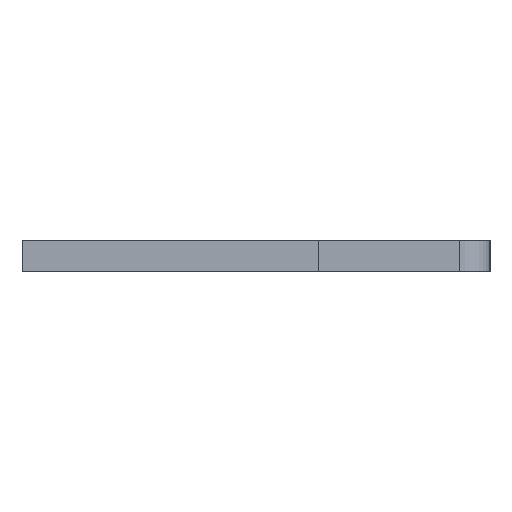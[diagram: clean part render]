
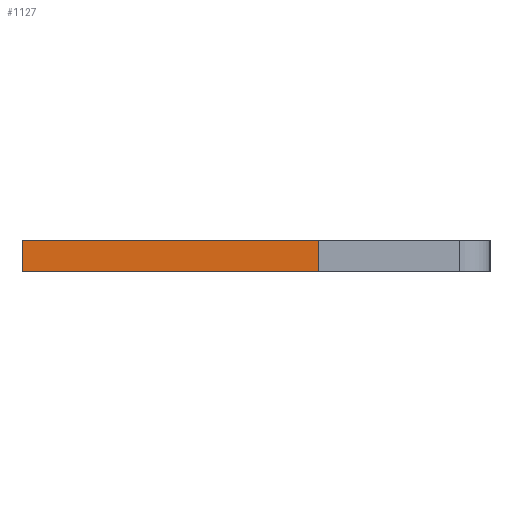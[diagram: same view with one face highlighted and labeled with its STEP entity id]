
A CAD part, left-side view. The second image highlights one B-rep face of the part: STEP entity #1127.
In plain terms, the highlighted face is planar.
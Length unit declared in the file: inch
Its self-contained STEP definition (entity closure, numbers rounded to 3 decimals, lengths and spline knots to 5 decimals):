
#14 = CARTESIAN_POINT ( 'NONE',  ( 0.01, 0.15, -0.04 ) ) ;
#43 = CARTESIAN_POINT ( 'NONE',  ( -0.01, -0.04, -0.04 ) ) ;
#54 = VECTOR ( 'NONE', #147, 39.37008 ) ;
#67 = EDGE_CURVE ( 'NONE', #194, #950, #928, .T. ) ;
#93 = EDGE_LOOP ( 'NONE', ( #683, #1497, #1712, #1092 ) ) ;
#97 = VECTOR ( 'NONE', #944, 39.37008 ) ;
#140 = CARTESIAN_POINT ( 'NONE',  ( -0.01, 0.15, -0.04 ) ) ;
#147 = DIRECTION ( 'NONE',  ( 0., 1., 0. ) ) ;
#194 = VERTEX_POINT ( 'NONE', #1778 ) ;
#210 = CARTESIAN_POINT ( 'NONE',  ( -0.01, 0.15, -0.04 ) ) ;
#486 = CARTESIAN_POINT ( 'NONE',  ( 0.01, -0.04, -0.04 ) ) ;
#551 = DIRECTION ( 'NONE',  ( 0., 1., 0. ) ) ;
#620 = VECTOR ( 'NONE', #884, 39.37008 ) ;
#644 = EDGE_CURVE ( 'NONE', #1469, #1506, #1287, .T. ) ;
#683 = ORIENTED_EDGE ( 'NONE', *, *, #644, .T. ) ;
#703 = EDGE_CURVE ( 'NONE', #950, #1506, #959, .T. ) ;
#875 = VECTOR ( 'NONE', #551, 39.37008 ) ;
#884 = DIRECTION ( 'NONE',  ( -1., 0., 0. ) ) ;
#891 = LINE ( 'NONE', #486, #97 ) ;
#894 = CARTESIAN_POINT ( 'NONE',  ( 0.01, 0.15, -0.04 ) ) ;
#928 = LINE ( 'NONE', #1938, #875 ) ;
#931 = DIRECTION ( 'NONE',  ( 0., 0., 1. ) ) ;
#944 = DIRECTION ( 'NONE',  ( -1., 0., 0. ) ) ;
#950 = VERTEX_POINT ( 'NONE', #1852 ) ;
#959 = LINE ( 'NONE', #894, #620 ) ;
#1092 = ORIENTED_EDGE ( 'NONE', *, *, #1315, .T. ) ;
#1127 = ADVANCED_FACE ( 'NONE', ( #1884 ), #1671, .F. ) ;
#1287 = LINE ( 'NONE', #140, #54 ) ;
#1315 = EDGE_CURVE ( 'NONE', #194, #1469, #891, .T. ) ;
#1323 = AXIS2_PLACEMENT_3D ( 'NONE', #14, #931, #1686 ) ;
#1469 = VERTEX_POINT ( 'NONE', #43 ) ;
#1497 = ORIENTED_EDGE ( 'NONE', *, *, #703, .F. ) ;
#1506 = VERTEX_POINT ( 'NONE', #210 ) ;
#1671 = PLANE ( 'NONE',  #1323 ) ;
#1686 = DIRECTION ( 'NONE',  ( 1., 0., 0. ) ) ;
#1712 = ORIENTED_EDGE ( 'NONE', *, *, #67, .F. ) ;
#1778 = CARTESIAN_POINT ( 'NONE',  ( 0.01, -0.04, -0.04 ) ) ;
#1852 = CARTESIAN_POINT ( 'NONE',  ( 0.01, 0.15, -0.04 ) ) ;
#1884 = FACE_OUTER_BOUND ( 'NONE', #93, .T. ) ;
#1938 = CARTESIAN_POINT ( 'NONE',  ( 0.01, 0.15, -0.04 ) ) ;
